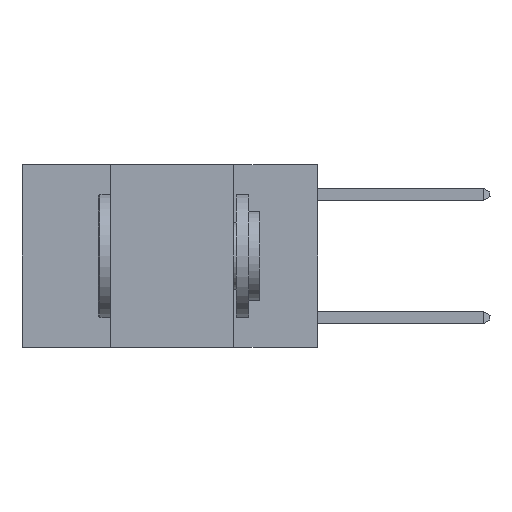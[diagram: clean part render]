
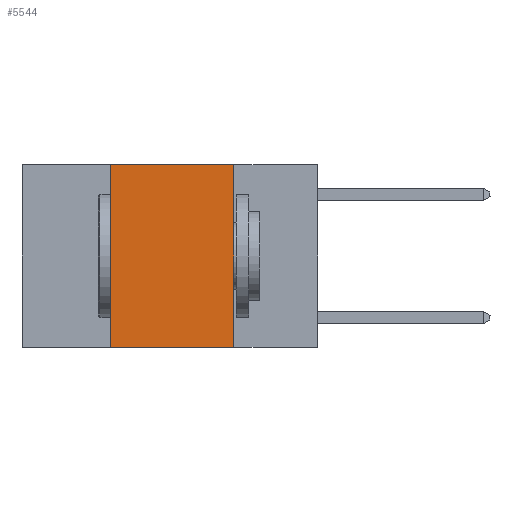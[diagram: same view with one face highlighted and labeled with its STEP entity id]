
A CAD part, left-side view. The second image highlights one B-rep face of the part: STEP entity #5544.
In plain terms, the highlighted planar face has unit normal (-1, 0, 0).
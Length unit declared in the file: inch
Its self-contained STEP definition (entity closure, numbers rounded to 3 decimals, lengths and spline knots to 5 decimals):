
#286 = CARTESIAN_POINT ( 'NONE',  ( 0., 0.42, 0. ) ) ;
#299 = LINE ( 'NONE', #7487, #1328 ) ;
#587 = EDGE_CURVE ( 'NONE', #9785, #2358, #299, .T. ) ;
#1328 = VECTOR ( 'NONE', #3013, 39.37008 ) ;
#1451 = VECTOR ( 'NONE', #2982, 39.37008 ) ;
#1674 = CARTESIAN_POINT ( 'NONE',  ( 0., 0.42, -0.37 ) ) ;
#2109 = CARTESIAN_POINT ( 'NONE',  ( 0., 0.42, 0. ) ) ;
#2185 = CARTESIAN_POINT ( 'NONE',  ( 0., 0.17, -0.37 ) ) ;
#2260 = VECTOR ( 'NONE', #10962, 39.37008 ) ;
#2358 = VERTEX_POINT ( 'NONE', #2185 ) ;
#2982 = DIRECTION ( 'NONE',  ( 0., 0., 1. ) ) ;
#2998 = VERTEX_POINT ( 'NONE', #1674 ) ;
#3013 = DIRECTION ( 'NONE',  ( 0., 0., -1. ) ) ;
#3145 = AXIS2_PLACEMENT_3D ( 'NONE', #5051, #4061, #11372 ) ;
#3981 = EDGE_LOOP ( 'NONE', ( #4245, #6119, #10897, #10710 ) ) ;
#4061 = DIRECTION ( 'NONE',  ( 1., 0., 0. ) ) ;
#4245 = ORIENTED_EDGE ( 'NONE', *, *, #587, .F. ) ;
#5051 = CARTESIAN_POINT ( 'NONE',  ( 0., 0.6, 0. ) ) ;
#5528 = EDGE_CURVE ( 'NONE', #8343, #9785, #5596, .T. ) ;
#5544 = ADVANCED_FACE ( 'NONE', ( #6572 ), #11124, .F. ) ;
#5596 = LINE ( 'NONE', #8277, #11542 ) ;
#6119 = ORIENTED_EDGE ( 'NONE', *, *, #5528, .F. ) ;
#6572 = FACE_OUTER_BOUND ( 'NONE', #3981, .T. ) ;
#6733 = EDGE_CURVE ( 'NONE', #2998, #8343, #9157, .T. ) ;
#7487 = CARTESIAN_POINT ( 'NONE',  ( 0., 0.17, 0. ) ) ;
#7566 = LINE ( 'NONE', #10095, #2260 ) ;
#8277 = CARTESIAN_POINT ( 'NONE',  ( 0., 0.6, 0. ) ) ;
#8343 = VERTEX_POINT ( 'NONE', #286 ) ;
#8390 = DIRECTION ( 'NONE',  ( 0., -1., 0. ) ) ;
#8964 = EDGE_CURVE ( 'NONE', #2998, #2358, #7566, .T. ) ;
#9121 = CARTESIAN_POINT ( 'NONE',  ( 0., 0.17, 0. ) ) ;
#9157 = LINE ( 'NONE', #2109, #1451 ) ;
#9785 = VERTEX_POINT ( 'NONE', #9121 ) ;
#10095 = CARTESIAN_POINT ( 'NONE',  ( 0., 0.6, -0.37 ) ) ;
#10710 = ORIENTED_EDGE ( 'NONE', *, *, #8964, .T. ) ;
#10897 = ORIENTED_EDGE ( 'NONE', *, *, #6733, .F. ) ;
#10962 = DIRECTION ( 'NONE',  ( 0., -1., 0. ) ) ;
#11124 = PLANE ( 'NONE',  #3145 ) ;
#11372 = DIRECTION ( 'NONE',  ( 0., 0., -1. ) ) ;
#11542 = VECTOR ( 'NONE', #8390, 39.37008 ) ;
